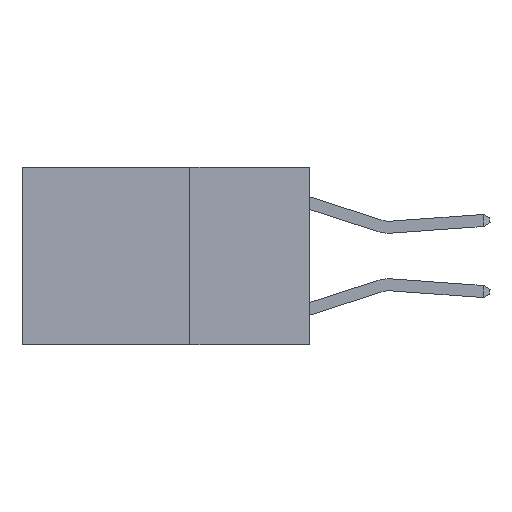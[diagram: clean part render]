
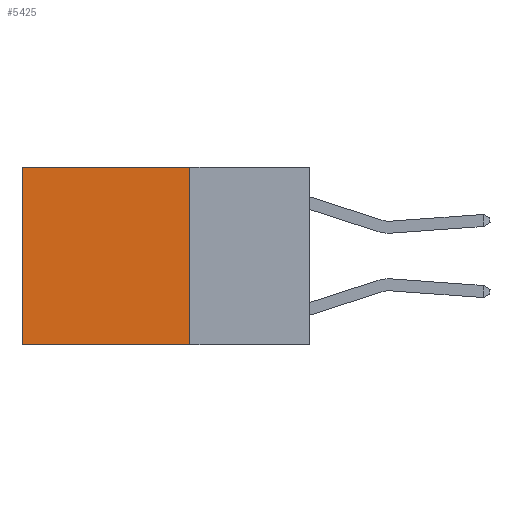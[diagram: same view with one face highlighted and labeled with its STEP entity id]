
A CAD part, left-side view. The second image highlights one B-rep face of the part: STEP entity #5425.
In plain terms, the highlighted planar face has unit normal (-1, 0, 0).
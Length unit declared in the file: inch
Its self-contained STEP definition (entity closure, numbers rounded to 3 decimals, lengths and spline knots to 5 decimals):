
#699 = AXIS2_PLACEMENT_3D ( 'NONE', #11052, #21886, #24236 ) ;
#881 = ORIENTED_EDGE ( 'NONE', *, *, #19743, .F. ) ;
#1496 = CARTESIAN_POINT ( 'NONE',  ( 0.2625, 0.6, -0.37 ) ) ;
#1595 = DIRECTION ( 'NONE',  ( 0., 0., -1. ) ) ;
#1816 = DIRECTION ( 'NONE',  ( 0., 0., -1. ) ) ;
#2791 = EDGE_CURVE ( 'NONE', #22212, #8352, #22479, .T. ) ;
#2924 = ORIENTED_EDGE ( 'NONE', *, *, #11546, .T. ) ;
#3059 = LINE ( 'NONE', #18091, #10541 ) ;
#3653 = CARTESIAN_POINT ( 'NONE',  ( 0.2625, 0.25, 0. ) ) ;
#4776 = VECTOR ( 'NONE', #1595, 39.37008 ) ;
#4903 = DIRECTION ( 'NONE',  ( 0., 1., 0. ) ) ;
#5425 = ADVANCED_FACE ( 'NONE', ( #11170 ), #18697, .F. ) ;
#8352 = VERTEX_POINT ( 'NONE', #9568 ) ;
#9202 = VERTEX_POINT ( 'NONE', #1496 ) ;
#9324 = ORIENTED_EDGE ( 'NONE', *, *, #24113, .T. ) ;
#9514 = EDGE_LOOP ( 'NONE', ( #2924, #881, #12070, #9324 ) ) ;
#9568 = CARTESIAN_POINT ( 'NONE',  ( 0.2625, 0.25, -0.37 ) ) ;
#10541 = VECTOR ( 'NONE', #4903, 39.37008 ) ;
#11052 = CARTESIAN_POINT ( 'NONE',  ( 0.2625, 0.25, 0. ) ) ;
#11170 = FACE_OUTER_BOUND ( 'NONE', #9514, .T. ) ;
#11546 = EDGE_CURVE ( 'NONE', #22561, #9202, #12544, .T. ) ;
#12070 = ORIENTED_EDGE ( 'NONE', *, *, #2791, .F. ) ;
#12298 = CARTESIAN_POINT ( 'NONE',  ( 0.2625, 0.6, 0. ) ) ;
#12544 = LINE ( 'NONE', #12298, #4776 ) ;
#13395 = LINE ( 'NONE', #20419, #16715 ) ;
#13944 = CARTESIAN_POINT ( 'NONE',  ( 0.2625, 0.25, 0. ) ) ;
#16715 = VECTOR ( 'NONE', #20776, 39.37008 ) ;
#17343 = CARTESIAN_POINT ( 'NONE',  ( 0.2625, 0.6, 0. ) ) ;
#18091 = CARTESIAN_POINT ( 'NONE',  ( 0.2625, 0.25, 0. ) ) ;
#18697 = PLANE ( 'NONE',  #699 ) ;
#19743 = EDGE_CURVE ( 'NONE', #8352, #9202, #13395, .T. ) ;
#20419 = CARTESIAN_POINT ( 'NONE',  ( 0.2625, 0.25, -0.37 ) ) ;
#20776 = DIRECTION ( 'NONE',  ( 0., 1., 0. ) ) ;
#21827 = VECTOR ( 'NONE', #1816, 39.37008 ) ;
#21886 = DIRECTION ( 'NONE',  ( 1., 0., 0. ) ) ;
#22212 = VERTEX_POINT ( 'NONE', #13944 ) ;
#22479 = LINE ( 'NONE', #3653, #21827 ) ;
#22561 = VERTEX_POINT ( 'NONE', #17343 ) ;
#24113 = EDGE_CURVE ( 'NONE', #22212, #22561, #3059, .T. ) ;
#24236 = DIRECTION ( 'NONE',  ( 0., 0., -1. ) ) ;
